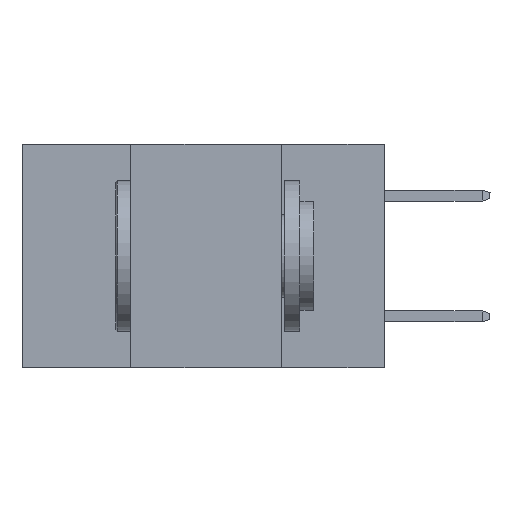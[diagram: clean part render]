
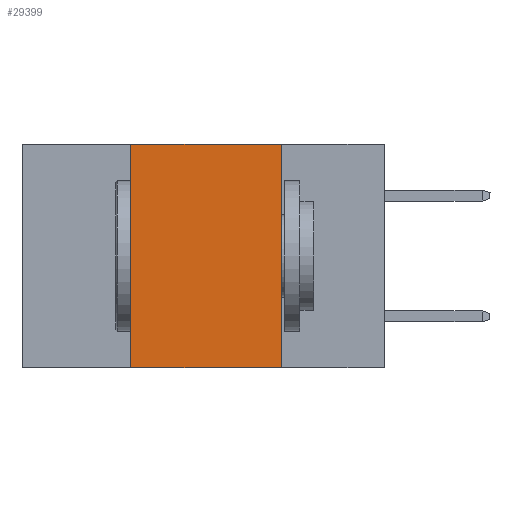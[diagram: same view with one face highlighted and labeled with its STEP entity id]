
A CAD part, left-side view. The second image highlights one B-rep face of the part: STEP entity #29399.
In plain terms, the highlighted planar face has unit normal (-1, 0, 0).
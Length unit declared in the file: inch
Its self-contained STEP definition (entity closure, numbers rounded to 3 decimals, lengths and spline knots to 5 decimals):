
#150 = CARTESIAN_POINT ( 'NONE',  ( 0., 0.6, 0. ) ) ;
#460 = EDGE_CURVE ( 'NONE', #32313, #10654, #12770, .T. ) ;
#688 = CARTESIAN_POINT ( 'NONE',  ( 0., 0.42, 0. ) ) ;
#1292 = VECTOR ( 'NONE', #30872, 39.37008 ) ;
#1956 = FACE_OUTER_BOUND ( 'NONE', #25262, .T. ) ;
#4205 = LINE ( 'NONE', #27623, #11996 ) ;
#4466 = ORIENTED_EDGE ( 'NONE', *, *, #460, .F. ) ;
#6564 = VECTOR ( 'NONE', #8819, 39.37008 ) ;
#7505 = DIRECTION ( 'NONE',  ( 0., 0., -1. ) ) ;
#8819 = DIRECTION ( 'NONE',  ( 0., 0., 1. ) ) ;
#9793 = DIRECTION ( 'NONE',  ( 0., -1., 0. ) ) ;
#10654 = VERTEX_POINT ( 'NONE', #688 ) ;
#11672 = EDGE_CURVE ( 'NONE', #21876, #24851, #32155, .T. ) ;
#11996 = VECTOR ( 'NONE', #33142, 39.37008 ) ;
#12770 = LINE ( 'NONE', #22197, #6564 ) ;
#13506 = CARTESIAN_POINT ( 'NONE',  ( 0., 0.42, -0.37 ) ) ;
#14513 = LINE ( 'NONE', #29967, #17834 ) ;
#17834 = VECTOR ( 'NONE', #9793, 39.37008 ) ;
#18197 = CARTESIAN_POINT ( 'NONE',  ( 0., 0.17, 0. ) ) ;
#18880 = EDGE_CURVE ( 'NONE', #10654, #21876, #4205, .T. ) ;
#19524 = ORIENTED_EDGE ( 'NONE', *, *, #11672, .F. ) ;
#21876 = VERTEX_POINT ( 'NONE', #18197 ) ;
#22197 = CARTESIAN_POINT ( 'NONE',  ( 0., 0.42, 0. ) ) ;
#23330 = DIRECTION ( 'NONE',  ( 1., 0., 0. ) ) ;
#24851 = VERTEX_POINT ( 'NONE', #34032 ) ;
#25262 = EDGE_LOOP ( 'NONE', ( #19524, #26330, #4466, #28274 ) ) ;
#25979 = AXIS2_PLACEMENT_3D ( 'NONE', #150, #23330, #7505 ) ;
#26330 = ORIENTED_EDGE ( 'NONE', *, *, #18880, .F. ) ;
#27623 = CARTESIAN_POINT ( 'NONE',  ( 0., 0.6, 0. ) ) ;
#28274 = ORIENTED_EDGE ( 'NONE', *, *, #33078, .T. ) ;
#29399 = ADVANCED_FACE ( 'NONE', ( #1956 ), #33970, .F. ) ;
#29967 = CARTESIAN_POINT ( 'NONE',  ( 0., 0.6, -0.37 ) ) ;
#30872 = DIRECTION ( 'NONE',  ( 0., 0., -1. ) ) ;
#30985 = CARTESIAN_POINT ( 'NONE',  ( 0., 0.17, 0. ) ) ;
#32155 = LINE ( 'NONE', #30985, #1292 ) ;
#32313 = VERTEX_POINT ( 'NONE', #13506 ) ;
#33078 = EDGE_CURVE ( 'NONE', #32313, #24851, #14513, .T. ) ;
#33142 = DIRECTION ( 'NONE',  ( 0., -1., 0. ) ) ;
#33970 = PLANE ( 'NONE',  #25979 ) ;
#34032 = CARTESIAN_POINT ( 'NONE',  ( 0., 0.17, -0.37 ) ) ;
